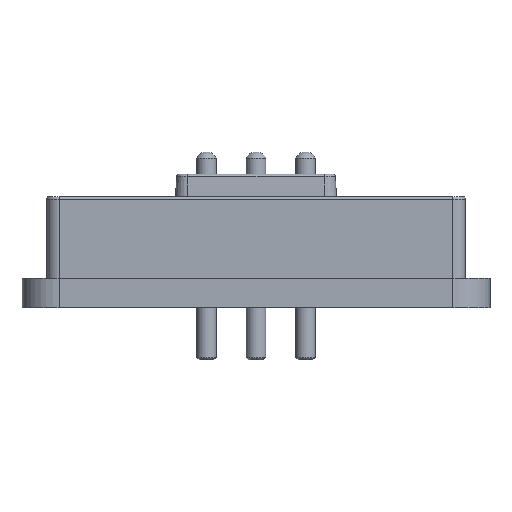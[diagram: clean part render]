
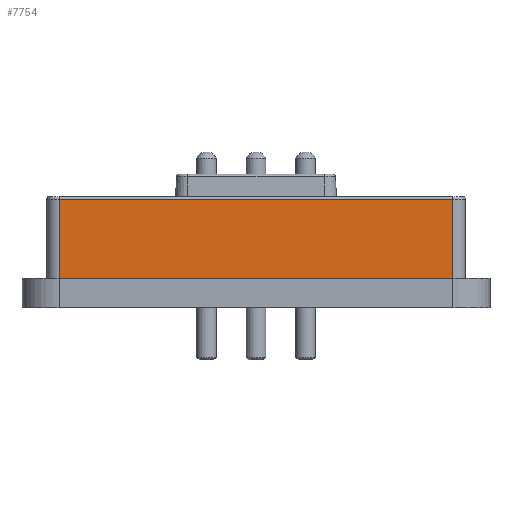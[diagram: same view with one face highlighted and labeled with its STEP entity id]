
A CAD part, front view. The second image highlights one B-rep face of the part: STEP entity #7754.
In plain terms, the highlighted planar face has unit normal (0, -1, 0).
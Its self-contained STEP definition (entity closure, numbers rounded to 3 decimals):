
#202 = CARTESIAN_POINT ( 'NONE',  ( -7.95, -2., -0.1 ) ) ;
#318 = CARTESIAN_POINT ( 'NONE',  ( 0., -2., -1.7 ) ) ;
#395 = EDGE_CURVE ( 'NONE', #2570, #9174, #8569, .T. ) ;
#581 = CARTESIAN_POINT ( 'NONE',  ( -7.95, -2., -3.3 ) ) ;
#944 = CARTESIAN_POINT ( 'NONE',  ( 7.95, -2., -3.3 ) ) ;
#1453 = ORIENTED_EDGE ( 'NONE', *, *, #10706, .T. ) ;
#2080 = VECTOR ( 'NONE', #3129, 1000. ) ;
#2106 = CARTESIAN_POINT ( 'NONE',  ( 7.95, -2., -0.1 ) ) ;
#2282 = EDGE_CURVE ( 'NONE', #9174, #9200, #2283, .T. ) ;
#2283 = LINE ( 'NONE', #9131, #4743 ) ;
#2565 = LINE ( 'NONE', #944, #9063 ) ;
#2570 = VERTEX_POINT ( 'NONE', #10050 ) ;
#3129 = DIRECTION ( 'NONE',  ( -1., 0., 0. ) ) ;
#3231 = ORIENTED_EDGE ( 'NONE', *, *, #2282, .T. ) ;
#4173 = DIRECTION ( 'NONE',  ( 0., 0., -1. ) ) ;
#4554 = FACE_OUTER_BOUND ( 'NONE', #6737, .T. ) ;
#4743 = VECTOR ( 'NONE', #4173, 1000. ) ;
#5179 = CARTESIAN_POINT ( 'NONE',  ( 7.95, -2., -3.3 ) ) ;
#5556 = CARTESIAN_POINT ( 'NONE',  ( -7.95, -2., -3.3 ) ) ;
#5828 = VECTOR ( 'NONE', #7121, 1000. ) ;
#5890 = ORIENTED_EDGE ( 'NONE', *, *, #395, .T. ) ;
#5925 = VERTEX_POINT ( 'NONE', #5179 ) ;
#6030 = DIRECTION ( 'NONE',  ( 0., 0., 1. ) ) ;
#6333 = DIRECTION ( 'NONE',  ( 0., 1., 0. ) ) ;
#6454 = PLANE ( 'NONE',  #11120 ) ;
#6737 = EDGE_LOOP ( 'NONE', ( #3231, #1453, #9863, #5890 ) ) ;
#7062 = DIRECTION ( 'NONE',  ( 1., 0., 0. ) ) ;
#7121 = DIRECTION ( 'NONE',  ( 1., 0., 0. ) ) ;
#7754 = ADVANCED_FACE ( 'NONE', ( #4554 ), #6454, .F. ) ;
#8569 = LINE ( 'NONE', #2106, #2080 ) ;
#9063 = VECTOR ( 'NONE', #6030, 1000. ) ;
#9131 = CARTESIAN_POINT ( 'NONE',  ( -7.95, -2., -0.1 ) ) ;
#9174 = VERTEX_POINT ( 'NONE', #202 ) ;
#9200 = VERTEX_POINT ( 'NONE', #581 ) ;
#9598 = EDGE_CURVE ( 'NONE', #5925, #2570, #2565, .T. ) ;
#9863 = ORIENTED_EDGE ( 'NONE', *, *, #9598, .T. ) ;
#10050 = CARTESIAN_POINT ( 'NONE',  ( 7.95, -2., -0.1 ) ) ;
#10635 = LINE ( 'NONE', #5556, #5828 ) ;
#10706 = EDGE_CURVE ( 'NONE', #9200, #5925, #10635, .T. ) ;
#11120 = AXIS2_PLACEMENT_3D ( 'NONE', #318, #6333, #7062 ) ;
